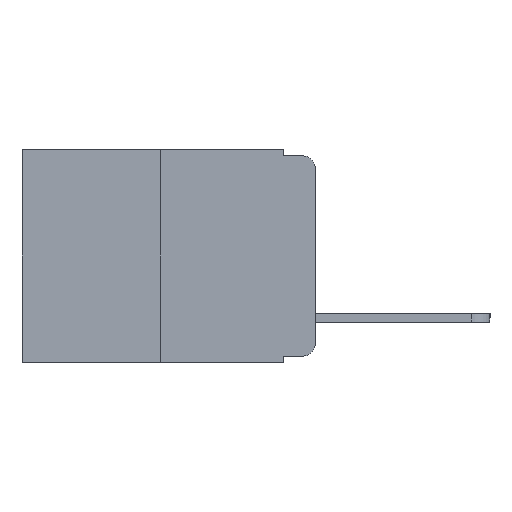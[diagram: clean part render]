
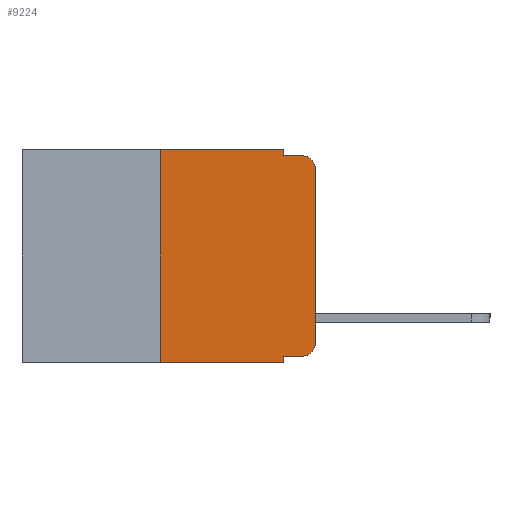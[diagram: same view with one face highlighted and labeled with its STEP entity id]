
A CAD part, left-side view. The second image highlights one B-rep face of the part: STEP entity #9224.
In plain terms, the highlighted planar face has unit normal (-1, 0, 0).
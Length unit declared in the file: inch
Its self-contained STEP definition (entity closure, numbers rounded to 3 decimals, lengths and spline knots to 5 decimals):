
#556 = DIRECTION ( 'NONE',  ( -1., 0., 0. ) ) ;
#637 = ORIENTED_EDGE ( 'NONE', *, *, #14224, .F. ) ;
#1363 = DIRECTION ( 'NONE',  ( 0., 0., -1. ) ) ;
#1434 = DIRECTION ( 'NONE',  ( 0., 0., -1. ) ) ;
#2002 = VERTEX_POINT ( 'NONE', #4852 ) ;
#2052 = EDGE_LOOP ( 'NONE', ( #2982, #16307, #3813, #637, #8123, #11708, #5481, #12095, #15747, #9671 ) ) ;
#2386 = VECTOR ( 'NONE', #10826, 39.37008 ) ;
#2409 = CARTESIAN_POINT ( 'NONE',  ( 0., 0.02, -0.01 ) ) ;
#2583 = DIRECTION ( 'NONE',  ( 0., 0., -1. ) ) ;
#2591 = LINE ( 'NONE', #11498, #15569 ) ;
#2860 = EDGE_CURVE ( 'NONE', #15842, #3272, #3891, .T. ) ;
#2982 = ORIENTED_EDGE ( 'NONE', *, *, #2860, .T. ) ;
#2996 = DIRECTION ( 'NONE',  ( 0., -1., 0. ) ) ;
#3272 = VERTEX_POINT ( 'NONE', #16404 ) ;
#3429 = EDGE_CURVE ( 'NONE', #8186, #5323, #14055, .T. ) ;
#3813 = ORIENTED_EDGE ( 'NONE', *, *, #4234, .F. ) ;
#3818 = FACE_OUTER_BOUND ( 'NONE', #2052, .T. ) ;
#3891 = LINE ( 'NONE', #8187, #10672 ) ;
#3997 = CARTESIAN_POINT ( 'NONE',  ( 0., 0.051, -0.01 ) ) ;
#4059 = LINE ( 'NONE', #13614, #13644 ) ;
#4234 = EDGE_CURVE ( 'NONE', #13375, #8386, #10252, .T. ) ;
#4450 = CARTESIAN_POINT ( 'NONE',  ( 0., 0.25, 0. ) ) ;
#4563 = VERTEX_POINT ( 'NONE', #11775 ) ;
#4652 = DIRECTION ( 'NONE',  ( 0., -1., 0. ) ) ;
#4852 = CARTESIAN_POINT ( 'NONE',  ( 0., 0.051, -0.343 ) ) ;
#5323 = VERTEX_POINT ( 'NONE', #13548 ) ;
#5365 = PLANE ( 'NONE',  #7513 ) ;
#5481 = ORIENTED_EDGE ( 'NONE', *, *, #15703, .T. ) ;
#5987 = CARTESIAN_POINT ( 'NONE',  ( 0., 0.051, -0.01 ) ) ;
#6328 = LINE ( 'NONE', #7086, #2386 ) ;
#6609 = CARTESIAN_POINT ( 'NONE',  ( 0., 0.473, 0. ) ) ;
#6916 = VECTOR ( 'NONE', #4652, 39.37008 ) ;
#7086 = CARTESIAN_POINT ( 'NONE',  ( 0., 0.25, 0. ) ) ;
#7513 = AXIS2_PLACEMENT_3D ( 'NONE', #6609, #9205, #1363 ) ;
#7795 = DIRECTION ( 'NONE',  ( -1., 0., 0. ) ) ;
#7799 = LINE ( 'NONE', #12853, #14264 ) ;
#8040 = EDGE_CURVE ( 'NONE', #4563, #15533, #6328, .T. ) ;
#8123 = ORIENTED_EDGE ( 'NONE', *, *, #13100, .F. ) ;
#8186 = VERTEX_POINT ( 'NONE', #12237 ) ;
#8187 = CARTESIAN_POINT ( 'NONE',  ( 0., 0., 0. ) ) ;
#8362 = VECTOR ( 'NONE', #2996, 39.37008 ) ;
#8386 = VERTEX_POINT ( 'NONE', #2409 ) ;
#8482 = CARTESIAN_POINT ( 'NONE',  ( 0., 0.02, -0.03 ) ) ;
#8678 = CARTESIAN_POINT ( 'NONE',  ( 0., 0.473, 0. ) ) ;
#9205 = DIRECTION ( 'NONE',  ( 1., 0., 0. ) ) ;
#9224 = ADVANCED_FACE ( 'NONE', ( #3818 ), #5365, .F. ) ;
#9671 = ORIENTED_EDGE ( 'NONE', *, *, #11968, .T. ) ;
#9735 = DIRECTION ( 'NONE',  ( 0., 0., -1. ) ) ;
#10017 = EDGE_CURVE ( 'NONE', #3272, #8386, #13973, .T. ) ;
#10059 = CARTESIAN_POINT ( 'NONE',  ( 0., 0., -0.313 ) ) ;
#10252 = LINE ( 'NONE', #5987, #6916 ) ;
#10662 = CARTESIAN_POINT ( 'NONE',  ( 0., 0.051, -0.333 ) ) ;
#10672 = VECTOR ( 'NONE', #15421, 39.37008 ) ;
#10826 = DIRECTION ( 'NONE',  ( 0., 0., 1. ) ) ;
#11306 = AXIS2_PLACEMENT_3D ( 'NONE', #8482, #556, #9735 ) ;
#11498 = CARTESIAN_POINT ( 'NONE',  ( 0., 0.051, 0. ) ) ;
#11708 = ORIENTED_EDGE ( 'NONE', *, *, #8040, .F. ) ;
#11775 = CARTESIAN_POINT ( 'NONE',  ( 0., 0.25, -0.343 ) ) ;
#11968 = EDGE_CURVE ( 'NONE', #5323, #15842, #15305, .T. ) ;
#12095 = ORIENTED_EDGE ( 'NONE', *, *, #15975, .F. ) ;
#12237 = CARTESIAN_POINT ( 'NONE',  ( 0., 0.051, -0.333 ) ) ;
#12853 = CARTESIAN_POINT ( 'NONE',  ( 0., 0.051, 0. ) ) ;
#13100 = EDGE_CURVE ( 'NONE', #15533, #14640, #13315, .T. ) ;
#13315 = LINE ( 'NONE', #8678, #16219 ) ;
#13375 = VERTEX_POINT ( 'NONE', #3997 ) ;
#13548 = CARTESIAN_POINT ( 'NONE',  ( 0., 0.02, -0.333 ) ) ;
#13614 = CARTESIAN_POINT ( 'NONE',  ( 0., 0.473, -0.343 ) ) ;
#13644 = VECTOR ( 'NONE', #14871, 39.37008 ) ;
#13973 = CIRCLE ( 'NONE', #11306, 0.02 ) ;
#14055 = LINE ( 'NONE', #10662, #8362 ) ;
#14224 = EDGE_CURVE ( 'NONE', #14640, #13375, #7799, .T. ) ;
#14264 = VECTOR ( 'NONE', #1434, 39.37008 ) ;
#14461 = AXIS2_PLACEMENT_3D ( 'NONE', #15094, #7795, #16314 ) ;
#14640 = VERTEX_POINT ( 'NONE', #14959 ) ;
#14871 = DIRECTION ( 'NONE',  ( 0., -1., 0. ) ) ;
#14959 = CARTESIAN_POINT ( 'NONE',  ( 0., 0.051, 0. ) ) ;
#15094 = CARTESIAN_POINT ( 'NONE',  ( 0., 0.02, -0.313 ) ) ;
#15305 = CIRCLE ( 'NONE', #14461, 0.02 ) ;
#15421 = DIRECTION ( 'NONE',  ( 0., 0., 1. ) ) ;
#15533 = VERTEX_POINT ( 'NONE', #4450 ) ;
#15569 = VECTOR ( 'NONE', #2583, 39.37008 ) ;
#15703 = EDGE_CURVE ( 'NONE', #4563, #2002, #4059, .T. ) ;
#15747 = ORIENTED_EDGE ( 'NONE', *, *, #3429, .T. ) ;
#15842 = VERTEX_POINT ( 'NONE', #10059 ) ;
#15955 = DIRECTION ( 'NONE',  ( 0., -1., 0. ) ) ;
#15975 = EDGE_CURVE ( 'NONE', #8186, #2002, #2591, .T. ) ;
#16219 = VECTOR ( 'NONE', #15955, 39.37008 ) ;
#16307 = ORIENTED_EDGE ( 'NONE', *, *, #10017, .T. ) ;
#16314 = DIRECTION ( 'NONE',  ( 0., 0., -1. ) ) ;
#16404 = CARTESIAN_POINT ( 'NONE',  ( 0., 0., -0.03 ) ) ;
